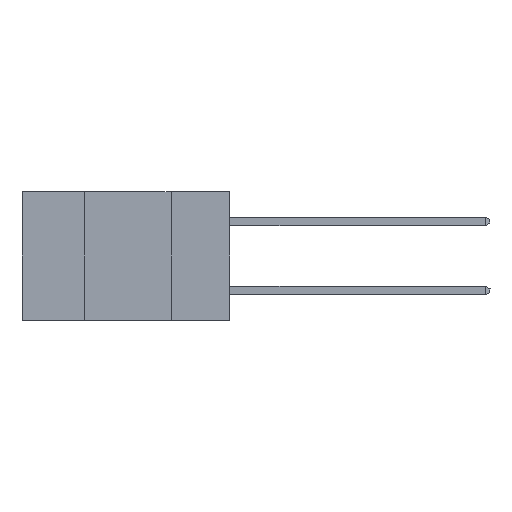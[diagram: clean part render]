
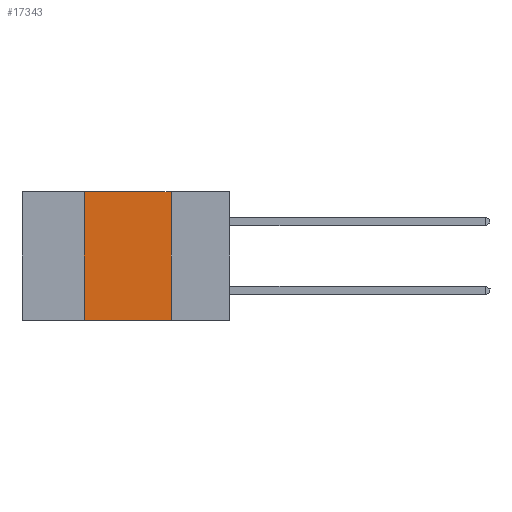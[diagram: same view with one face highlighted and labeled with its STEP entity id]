
A CAD part, left-side view. The second image highlights one B-rep face of the part: STEP entity #17343.
In plain terms, the highlighted planar face has unit normal (-1, 0, 0).
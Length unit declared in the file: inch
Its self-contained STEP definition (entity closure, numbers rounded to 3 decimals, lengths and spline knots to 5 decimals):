
#80 = EDGE_CURVE ( 'NONE', #1097, #1543, #21561, .T. ) ;
#501 = EDGE_LOOP ( 'NONE', ( #10499, #18895, #19667, #13526 ) ) ;
#612 = LINE ( 'NONE', #4215, #13716 ) ;
#1097 = VERTEX_POINT ( 'NONE', #8104 ) ;
#1543 = VERTEX_POINT ( 'NONE', #6473 ) ;
#1750 = LINE ( 'NONE', #6249, #22028 ) ;
#2040 = EDGE_CURVE ( 'NONE', #1543, #14059, #1750, .T. ) ;
#3025 = EDGE_CURVE ( 'NONE', #14059, #19979, #3868, .T. ) ;
#3300 = DIRECTION ( 'NONE',  ( 0., 0., 1. ) ) ;
#3868 = LINE ( 'NONE', #15563, #6783 ) ;
#4215 = CARTESIAN_POINT ( 'NONE',  ( 0., 0.6, -0.37 ) ) ;
#4693 = CARTESIAN_POINT ( 'NONE',  ( 0., 0.17, -0.37 ) ) ;
#4707 = PLANE ( 'NONE',  #18058 ) ;
#6249 = CARTESIAN_POINT ( 'NONE',  ( 0., 0.6, 0. ) ) ;
#6473 = CARTESIAN_POINT ( 'NONE',  ( 0., 0.42, 0. ) ) ;
#6783 = VECTOR ( 'NONE', #15709, 39.37008 ) ;
#7891 = CARTESIAN_POINT ( 'NONE',  ( 0., 0.6, 0. ) ) ;
#8104 = CARTESIAN_POINT ( 'NONE',  ( 0., 0.42, -0.37 ) ) ;
#8258 = CARTESIAN_POINT ( 'NONE',  ( 0., 0.42, 0. ) ) ;
#10499 = ORIENTED_EDGE ( 'NONE', *, *, #3025, .F. ) ;
#12774 = DIRECTION ( 'NONE',  ( 0., -1., 0. ) ) ;
#13286 = CARTESIAN_POINT ( 'NONE',  ( 0., 0.17, 0. ) ) ;
#13526 = ORIENTED_EDGE ( 'NONE', *, *, #17200, .T. ) ;
#13716 = VECTOR ( 'NONE', #12774, 39.37008 ) ;
#14059 = VERTEX_POINT ( 'NONE', #13286 ) ;
#14692 = DIRECTION ( 'NONE',  ( 0., -1., 0. ) ) ;
#14928 = DIRECTION ( 'NONE',  ( 0., 0., -1. ) ) ;
#15563 = CARTESIAN_POINT ( 'NONE',  ( 0., 0.17, 0. ) ) ;
#15709 = DIRECTION ( 'NONE',  ( 0., 0., -1. ) ) ;
#16562 = DIRECTION ( 'NONE',  ( 1., 0., 0. ) ) ;
#17200 = EDGE_CURVE ( 'NONE', #1097, #19979, #612, .T. ) ;
#17343 = ADVANCED_FACE ( 'NONE', ( #18805 ), #4707, .F. ) ;
#18058 = AXIS2_PLACEMENT_3D ( 'NONE', #7891, #16562, #14928 ) ;
#18653 = VECTOR ( 'NONE', #3300, 39.37008 ) ;
#18805 = FACE_OUTER_BOUND ( 'NONE', #501, .T. ) ;
#18895 = ORIENTED_EDGE ( 'NONE', *, *, #2040, .F. ) ;
#19667 = ORIENTED_EDGE ( 'NONE', *, *, #80, .F. ) ;
#19979 = VERTEX_POINT ( 'NONE', #4693 ) ;
#21561 = LINE ( 'NONE', #8258, #18653 ) ;
#22028 = VECTOR ( 'NONE', #14692, 39.37008 ) ;
